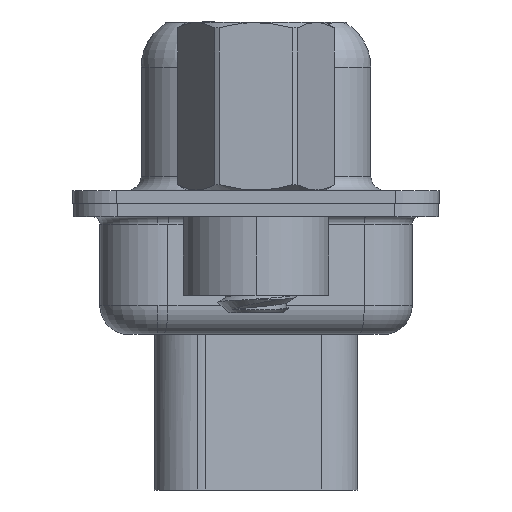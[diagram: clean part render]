
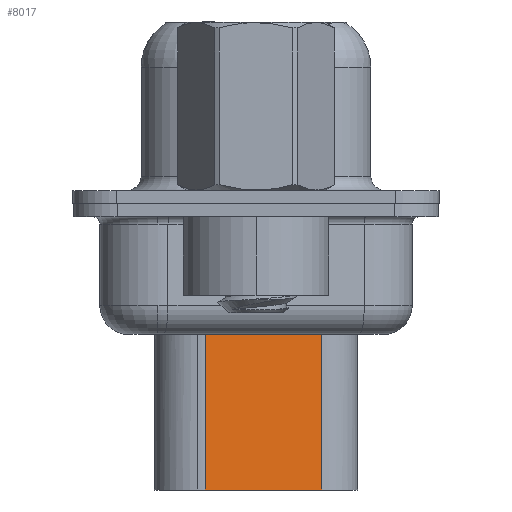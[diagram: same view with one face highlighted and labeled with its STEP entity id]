
A CAD part, left-side view. The second image highlights one B-rep face of the part: STEP entity #8017.
In plain terms, the highlighted planar face has unit normal (-0.985, -0.174, 0).
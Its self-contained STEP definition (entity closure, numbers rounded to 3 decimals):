
#89 = CARTESIAN_POINT ( 'NONE',  ( 5.214, -2.26, -9.85 ) ) ;
#1458 = EDGE_CURVE ( 'NONE', #10710, #16928, #18243, .T. ) ;
#2027 = CARTESIAN_POINT ( 'NONE',  ( 4.338, 2.709, -3.975 ) ) ;
#2402 = CARTESIAN_POINT ( 'NONE',  ( 4.509, 1.74, -3.1 ) ) ;
#2903 = VECTOR ( 'NONE', #11450, 1000. ) ;
#3341 = PLANE ( 'NONE',  #10030 ) ;
#4176 = CARTESIAN_POINT ( 'NONE',  ( 5.214, -2.26, -3.1 ) ) ;
#4180 = CARTESIAN_POINT ( 'NONE',  ( 4.509, 1.74, -3.975 ) ) ;
#4353 = VECTOR ( 'NONE', #16208, 1000. ) ;
#5269 = EDGE_CURVE ( 'NONE', #10710, #13102, #22298, .T. ) ;
#5787 = EDGE_LOOP ( 'NONE', ( #7489, #20815, #19556, #22238 ) ) ;
#5974 = LINE ( 'NONE', #2402, #18042 ) ;
#7489 = ORIENTED_EDGE ( 'NONE', *, *, #5269, .F. ) ;
#8017 = ADVANCED_FACE ( 'NONE', ( #22060 ), #3341, .T. ) ;
#9180 = CARTESIAN_POINT ( 'NONE',  ( 4.509, 1.74, -3.1 ) ) ;
#10030 = AXIS2_PLACEMENT_3D ( 'NONE', #9180, #16091, #10741 ) ;
#10710 = VERTEX_POINT ( 'NONE', #11804 ) ;
#10741 = DIRECTION ( 'NONE',  ( 0.174, -0.985, 0. ) ) ;
#11450 = DIRECTION ( 'NONE',  ( 0., 0., -1. ) ) ;
#11804 = CARTESIAN_POINT ( 'NONE',  ( 5.214, -2.26, -3.975 ) ) ;
#12911 = DIRECTION ( 'NONE',  ( 0., 0., -1. ) ) ;
#13102 = VERTEX_POINT ( 'NONE', #89 ) ;
#13628 = CARTESIAN_POINT ( 'NONE',  ( 4.509, 1.74, -9.85 ) ) ;
#13889 = EDGE_CURVE ( 'NONE', #16928, #20786, #5974, .T. ) ;
#15566 = EDGE_CURVE ( 'NONE', #13102, #20786, #21256, .T. ) ;
#15992 = DIRECTION ( 'NONE',  ( -0.174, 0.985, 0. ) ) ;
#16091 = DIRECTION ( 'NONE',  ( -0.985, -0.174, 0. ) ) ;
#16208 = DIRECTION ( 'NONE',  ( -0.174, 0.985, 0. ) ) ;
#16928 = VERTEX_POINT ( 'NONE', #4180 ) ;
#18042 = VECTOR ( 'NONE', #12911, 1000. ) ;
#18243 = LINE ( 'NONE', #2027, #4353 ) ;
#19556 = ORIENTED_EDGE ( 'NONE', *, *, #13889, .T. ) ;
#20786 = VERTEX_POINT ( 'NONE', #13628 ) ;
#20815 = ORIENTED_EDGE ( 'NONE', *, *, #1458, .T. ) ;
#21140 = CARTESIAN_POINT ( 'NONE',  ( 4.509, 1.74, -9.85 ) ) ;
#21256 = LINE ( 'NONE', #21140, #22694 ) ;
#22060 = FACE_OUTER_BOUND ( 'NONE', #5787, .T. ) ;
#22238 = ORIENTED_EDGE ( 'NONE', *, *, #15566, .F. ) ;
#22298 = LINE ( 'NONE', #4176, #2903 ) ;
#22694 = VECTOR ( 'NONE', #15992, 1000. ) ;
